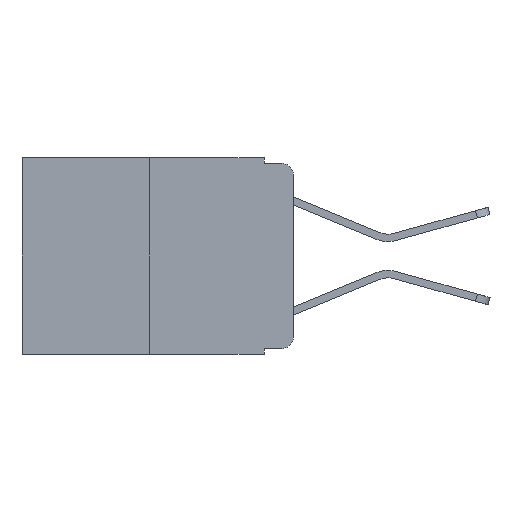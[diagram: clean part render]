
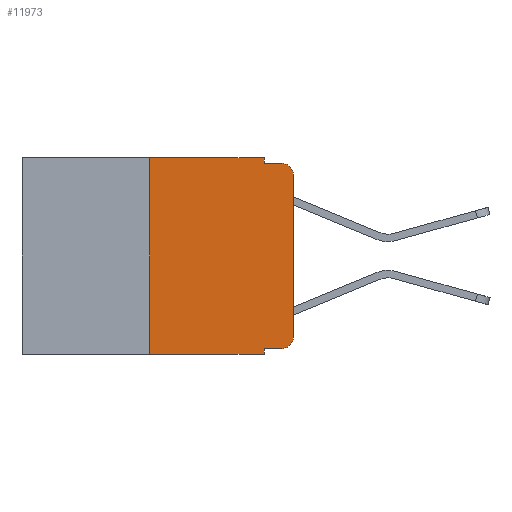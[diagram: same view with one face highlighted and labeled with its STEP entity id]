
A CAD part, left-side view. The second image highlights one B-rep face of the part: STEP entity #11973.
In plain terms, the highlighted planar face has unit normal (-1, 0, 0).
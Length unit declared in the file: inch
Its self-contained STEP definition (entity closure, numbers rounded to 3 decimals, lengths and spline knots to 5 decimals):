
#95 = EDGE_CURVE ( 'NONE', #6325, #3463, #2143, .T. ) ;
#263 = AXIS2_PLACEMENT_3D ( 'NONE', #11983, #5032, #3852 ) ;
#534 = EDGE_CURVE ( 'NONE', #10243, #3463, #10205, .T. ) ;
#680 = FACE_OUTER_BOUND ( 'NONE', #17381, .T. ) ;
#974 = EDGE_CURVE ( 'NONE', #7956, #15019, #9975, .T. ) ;
#1116 = PLANE ( 'NONE',  #263 ) ;
#1400 = AXIS2_PLACEMENT_3D ( 'NONE', #9779, #8182, #8242 ) ;
#1486 = ORIENTED_EDGE ( 'NONE', *, *, #3181, .F. ) ;
#1768 = EDGE_CURVE ( 'NONE', #7990, #3504, #5675, .T. ) ;
#1827 = DIRECTION ( 'NONE',  ( -1., 0., 0. ) ) ;
#2143 = LINE ( 'NONE', #14701, #16124 ) ;
#2300 = DIRECTION ( 'NONE',  ( 0., -1., 0. ) ) ;
#2730 = CARTESIAN_POINT ( 'NONE',  ( 0., 0.051, -0.01 ) ) ;
#2859 = VECTOR ( 'NONE', #12875, 39.37008 ) ;
#3181 = EDGE_CURVE ( 'NONE', #6325, #5592, #16017, .T. ) ;
#3197 = CARTESIAN_POINT ( 'NONE',  ( 0., 0.02, -0.03 ) ) ;
#3463 = VERTEX_POINT ( 'NONE', #3866 ) ;
#3504 = VERTEX_POINT ( 'NONE', #16166 ) ;
#3852 = DIRECTION ( 'NONE',  ( 0., 0., -1. ) ) ;
#3866 = CARTESIAN_POINT ( 'NONE',  ( 0., 0.051, -0.343 ) ) ;
#3882 = ORIENTED_EDGE ( 'NONE', *, *, #534, .F. ) ;
#4043 = DIRECTION ( 'NONE',  ( 0., -1., 0. ) ) ;
#4364 = CARTESIAN_POINT ( 'NONE',  ( 0., 0., 0. ) ) ;
#4574 = CARTESIAN_POINT ( 'NONE',  ( 0., 0.473, 0. ) ) ;
#4699 = ORIENTED_EDGE ( 'NONE', *, *, #95, .T. ) ;
#5032 = DIRECTION ( 'NONE',  ( 1., 0., 0. ) ) ;
#5438 = CARTESIAN_POINT ( 'NONE',  ( 0., 0.051, 0. ) ) ;
#5592 = VERTEX_POINT ( 'NONE', #9266 ) ;
#5675 = LINE ( 'NONE', #4364, #7808 ) ;
#5780 = EDGE_CURVE ( 'NONE', #14033, #7990, #6373, .T. ) ;
#6011 = DIRECTION ( 'NONE',  ( 0., 0., 1. ) ) ;
#6322 = CARTESIAN_POINT ( 'NONE',  ( 0., 0.02, -0.01 ) ) ;
#6325 = VERTEX_POINT ( 'NONE', #17139 ) ;
#6373 = CIRCLE ( 'NONE', #1400, 0.02 ) ;
#6491 = ORIENTED_EDGE ( 'NONE', *, *, #9970, .F. ) ;
#6575 = VECTOR ( 'NONE', #13085, 39.37008 ) ;
#7285 = DIRECTION ( 'NONE',  ( 0., 0., -1. ) ) ;
#7765 = VECTOR ( 'NONE', #6011, 39.37008 ) ;
#7808 = VECTOR ( 'NONE', #11132, 39.37008 ) ;
#7956 = VERTEX_POINT ( 'NONE', #8552 ) ;
#7990 = VERTEX_POINT ( 'NONE', #12502 ) ;
#7995 = CARTESIAN_POINT ( 'NONE',  ( 0., 0.051, -0.333 ) ) ;
#8182 = DIRECTION ( 'NONE',  ( -1., 0., 0. ) ) ;
#8242 = DIRECTION ( 'NONE',  ( 0., 0., -1. ) ) ;
#8259 = VECTOR ( 'NONE', #2300, 39.37008 ) ;
#8392 = DIRECTION ( 'NONE',  ( 0., -1., 0. ) ) ;
#8514 = CARTESIAN_POINT ( 'NONE',  ( 0., 0.25, 0. ) ) ;
#8552 = CARTESIAN_POINT ( 'NONE',  ( 0., 0.051, -0.01 ) ) ;
#8622 = CARTESIAN_POINT ( 'NONE',  ( 0., 0.051, 0. ) ) ;
#8920 = ORIENTED_EDGE ( 'NONE', *, *, #5780, .T. ) ;
#9266 = CARTESIAN_POINT ( 'NONE',  ( 0., 0.25, 0. ) ) ;
#9647 = VERTEX_POINT ( 'NONE', #5438 ) ;
#9779 = CARTESIAN_POINT ( 'NONE',  ( 0., 0.02, -0.313 ) ) ;
#9970 = EDGE_CURVE ( 'NONE', #9647, #7956, #13856, .T. ) ;
#9975 = LINE ( 'NONE', #2730, #8259 ) ;
#10084 = LINE ( 'NONE', #11530, #2859 ) ;
#10205 = LINE ( 'NONE', #11752, #6575 ) ;
#10243 = VERTEX_POINT ( 'NONE', #7995 ) ;
#10514 = CARTESIAN_POINT ( 'NONE',  ( 0., 0.02, -0.333 ) ) ;
#10578 = ORIENTED_EDGE ( 'NONE', *, *, #12388, .T. ) ;
#11047 = CIRCLE ( 'NONE', #15473, 0.02 ) ;
#11132 = DIRECTION ( 'NONE',  ( 0., 0., 1. ) ) ;
#11530 = CARTESIAN_POINT ( 'NONE',  ( 0., 0.051, -0.333 ) ) ;
#11752 = CARTESIAN_POINT ( 'NONE',  ( 0., 0.051, 0. ) ) ;
#11973 = ADVANCED_FACE ( 'NONE', ( #680 ), #1116, .F. ) ;
#11983 = CARTESIAN_POINT ( 'NONE',  ( 0., 0.473, 0. ) ) ;
#12310 = ORIENTED_EDGE ( 'NONE', *, *, #974, .F. ) ;
#12388 = EDGE_CURVE ( 'NONE', #3504, #15019, #11047, .T. ) ;
#12409 = LINE ( 'NONE', #4574, #12630 ) ;
#12502 = CARTESIAN_POINT ( 'NONE',  ( 0., 0., -0.313 ) ) ;
#12630 = VECTOR ( 'NONE', #8392, 39.37008 ) ;
#12875 = DIRECTION ( 'NONE',  ( 0., -1., 0. ) ) ;
#13085 = DIRECTION ( 'NONE',  ( 0., 0., -1. ) ) ;
#13856 = LINE ( 'NONE', #8622, #16846 ) ;
#14033 = VERTEX_POINT ( 'NONE', #10514 ) ;
#14701 = CARTESIAN_POINT ( 'NONE',  ( 0., 0.473, -0.343 ) ) ;
#14785 = ORIENTED_EDGE ( 'NONE', *, *, #1768, .T. ) ;
#15019 = VERTEX_POINT ( 'NONE', #6322 ) ;
#15433 = EDGE_CURVE ( 'NONE', #5592, #9647, #12409, .T. ) ;
#15456 = DIRECTION ( 'NONE',  ( 0., 0., -1. ) ) ;
#15473 = AXIS2_PLACEMENT_3D ( 'NONE', #3197, #1827, #15456 ) ;
#15674 = EDGE_CURVE ( 'NONE', #10243, #14033, #10084, .T. ) ;
#16017 = LINE ( 'NONE', #8514, #7765 ) ;
#16124 = VECTOR ( 'NONE', #4043, 39.37008 ) ;
#16166 = CARTESIAN_POINT ( 'NONE',  ( 0., 0., -0.03 ) ) ;
#16416 = ORIENTED_EDGE ( 'NONE', *, *, #15674, .T. ) ;
#16846 = VECTOR ( 'NONE', #7285, 39.37008 ) ;
#17139 = CARTESIAN_POINT ( 'NONE',  ( 0., 0.25, -0.343 ) ) ;
#17381 = EDGE_LOOP ( 'NONE', ( #14785, #10578, #12310, #6491, #17402, #1486, #4699, #3882, #16416, #8920 ) ) ;
#17402 = ORIENTED_EDGE ( 'NONE', *, *, #15433, .F. ) ;
